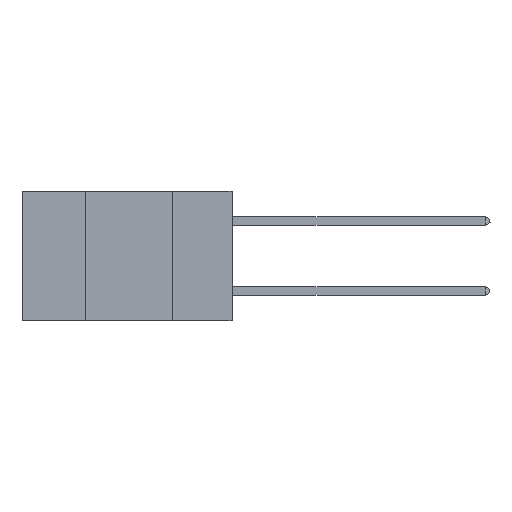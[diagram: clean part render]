
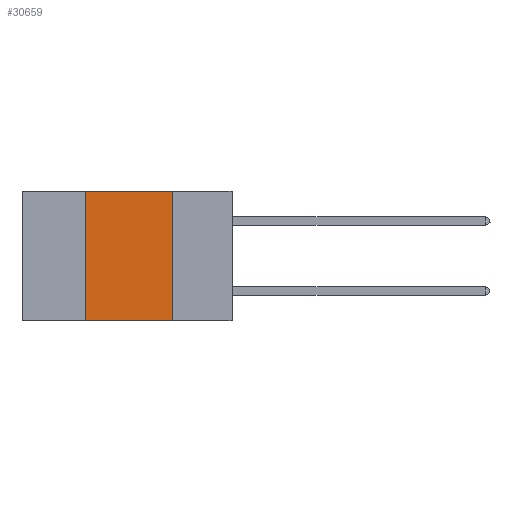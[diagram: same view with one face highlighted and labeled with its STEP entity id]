
A CAD part, left-side view. The second image highlights one B-rep face of the part: STEP entity #30659.
In plain terms, the highlighted planar face has unit normal (-1, 0, 0).
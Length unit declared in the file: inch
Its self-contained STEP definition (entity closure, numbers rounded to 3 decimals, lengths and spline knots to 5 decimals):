
#1315 = ORIENTED_EDGE ( 'NONE', *, *, #23468, .T. ) ;
#2353 = ORIENTED_EDGE ( 'NONE', *, *, #17352, .F. ) ;
#2530 = CARTESIAN_POINT ( 'NONE',  ( 0., 0.17, 0. ) ) ;
#3006 = VERTEX_POINT ( 'NONE', #6553 ) ;
#5458 = LINE ( 'NONE', #11253, #40020 ) ;
#6553 = CARTESIAN_POINT ( 'NONE',  ( 0., 0.42, 0. ) ) ;
#7187 = DIRECTION ( 'NONE',  ( 0., -1., 0. ) ) ;
#7694 = ORIENTED_EDGE ( 'NONE', *, *, #22455, .F. ) ;
#9854 = AXIS2_PLACEMENT_3D ( 'NONE', #13629, #30348, #10404 ) ;
#10404 = DIRECTION ( 'NONE',  ( 0., 0., -1. ) ) ;
#10599 = CARTESIAN_POINT ( 'NONE',  ( 0., 0.6, -0.37 ) ) ;
#11253 = CARTESIAN_POINT ( 'NONE',  ( 0., 0.42, 0. ) ) ;
#11455 = EDGE_CURVE ( 'NONE', #33100, #3006, #5458, .T. ) ;
#11543 = DIRECTION ( 'NONE',  ( 0., 0., 1. ) ) ;
#12446 = DIRECTION ( 'NONE',  ( 0., -1., 0. ) ) ;
#13629 = CARTESIAN_POINT ( 'NONE',  ( 0., 0.6, 0. ) ) ;
#17352 = EDGE_CURVE ( 'NONE', #23955, #39305, #29157, .T. ) ;
#20390 = EDGE_LOOP ( 'NONE', ( #2353, #7694, #39589, #1315 ) ) ;
#22455 = EDGE_CURVE ( 'NONE', #3006, #23955, #29081, .T. ) ;
#23468 = EDGE_CURVE ( 'NONE', #33100, #39305, #31582, .T. ) ;
#23955 = VERTEX_POINT ( 'NONE', #39608 ) ;
#27043 = PLANE ( 'NONE',  #9854 ) ;
#29081 = LINE ( 'NONE', #35759, #37981 ) ;
#29157 = LINE ( 'NONE', #2530, #37028 ) ;
#29325 = DIRECTION ( 'NONE',  ( 0., 0., -1. ) ) ;
#30348 = DIRECTION ( 'NONE',  ( 1., 0., 0. ) ) ;
#30546 = VECTOR ( 'NONE', #7187, 39.37008 ) ;
#30659 = ADVANCED_FACE ( 'NONE', ( #31448 ), #27043, .F. ) ;
#31448 = FACE_OUTER_BOUND ( 'NONE', #20390, .T. ) ;
#31582 = LINE ( 'NONE', #10599, #30546 ) ;
#33100 = VERTEX_POINT ( 'NONE', #35020 ) ;
#35020 = CARTESIAN_POINT ( 'NONE',  ( 0., 0.42, -0.37 ) ) ;
#35759 = CARTESIAN_POINT ( 'NONE',  ( 0., 0.6, 0. ) ) ;
#37028 = VECTOR ( 'NONE', #29325, 39.37008 ) ;
#37981 = VECTOR ( 'NONE', #12446, 39.37008 ) ;
#39305 = VERTEX_POINT ( 'NONE', #40004 ) ;
#39589 = ORIENTED_EDGE ( 'NONE', *, *, #11455, .F. ) ;
#39608 = CARTESIAN_POINT ( 'NONE',  ( 0., 0.17, 0. ) ) ;
#40004 = CARTESIAN_POINT ( 'NONE',  ( 0., 0.17, -0.37 ) ) ;
#40020 = VECTOR ( 'NONE', #11543, 39.37008 ) ;
